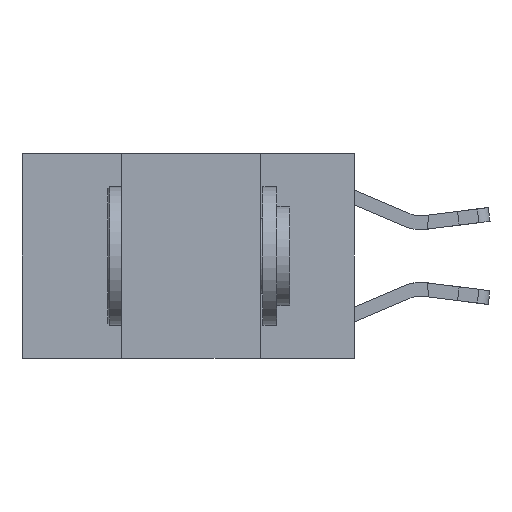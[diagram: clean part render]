
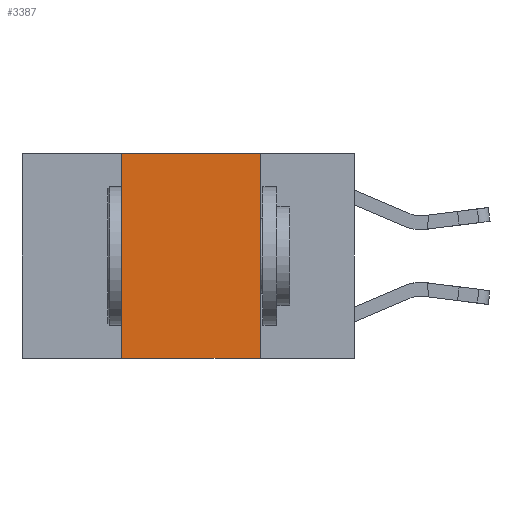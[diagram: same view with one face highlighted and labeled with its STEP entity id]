
A CAD part, left-side view. The second image highlights one B-rep face of the part: STEP entity #3387.
In plain terms, the highlighted planar face has unit normal (-1, 0, 0).
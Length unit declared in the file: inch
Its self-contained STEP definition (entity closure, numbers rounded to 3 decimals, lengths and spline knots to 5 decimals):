
#477 = VERTEX_POINT ( 'NONE', #1706 ) ;
#646 = EDGE_CURVE ( 'NONE', #9966, #10635, #1362, .T. ) ;
#949 = EDGE_CURVE ( 'NONE', #477, #2112, #10585, .T. ) ;
#1362 = LINE ( 'NONE', #8092, #7666 ) ;
#1706 = CARTESIAN_POINT ( 'NONE',  ( 0., 0.17, 0. ) ) ;
#1920 = CARTESIAN_POINT ( 'NONE',  ( 0., 0.6, -0.37 ) ) ;
#1939 = VECTOR ( 'NONE', #5549, 39.37008 ) ;
#2112 = VERTEX_POINT ( 'NONE', #10304 ) ;
#2178 = EDGE_CURVE ( 'NONE', #10635, #477, #13359, .T. ) ;
#2293 = LINE ( 'NONE', #1920, #1939 ) ;
#3252 = AXIS2_PLACEMENT_3D ( 'NONE', #7970, #13397, #6869 ) ;
#3387 = ADVANCED_FACE ( 'NONE', ( #7974 ), #5745, .F. ) ;
#4609 = CARTESIAN_POINT ( 'NONE',  ( 0., 0.42, -0.37 ) ) ;
#5238 = ORIENTED_EDGE ( 'NONE', *, *, #7567, .T. ) ;
#5549 = DIRECTION ( 'NONE',  ( 0., -1., 0. ) ) ;
#5692 = VECTOR ( 'NONE', #5843, 39.37008 ) ;
#5745 = PLANE ( 'NONE',  #3252 ) ;
#5843 = DIRECTION ( 'NONE',  ( 0., 0., -1. ) ) ;
#6869 = DIRECTION ( 'NONE',  ( 0., 0., -1. ) ) ;
#7567 = EDGE_CURVE ( 'NONE', #9966, #2112, #2293, .T. ) ;
#7666 = VECTOR ( 'NONE', #8323, 39.37008 ) ;
#7970 = CARTESIAN_POINT ( 'NONE',  ( 0., 0.6, 0. ) ) ;
#7974 = FACE_OUTER_BOUND ( 'NONE', #13854, .T. ) ;
#8092 = CARTESIAN_POINT ( 'NONE',  ( 0., 0.42, 0. ) ) ;
#8323 = DIRECTION ( 'NONE',  ( 0., 0., 1. ) ) ;
#9466 = ORIENTED_EDGE ( 'NONE', *, *, #646, .F. ) ;
#9500 = CARTESIAN_POINT ( 'NONE',  ( 0., 0.17, 0. ) ) ;
#9966 = VERTEX_POINT ( 'NONE', #4609 ) ;
#10304 = CARTESIAN_POINT ( 'NONE',  ( 0., 0.17, -0.37 ) ) ;
#10547 = VECTOR ( 'NONE', #12712, 39.37008 ) ;
#10584 = CARTESIAN_POINT ( 'NONE',  ( 0., 0.6, 0. ) ) ;
#10585 = LINE ( 'NONE', #9500, #5692 ) ;
#10635 = VERTEX_POINT ( 'NONE', #11976 ) ;
#11955 = ORIENTED_EDGE ( 'NONE', *, *, #949, .F. ) ;
#11976 = CARTESIAN_POINT ( 'NONE',  ( 0., 0.42, 0. ) ) ;
#12435 = ORIENTED_EDGE ( 'NONE', *, *, #2178, .F. ) ;
#12712 = DIRECTION ( 'NONE',  ( 0., -1., 0. ) ) ;
#13359 = LINE ( 'NONE', #10584, #10547 ) ;
#13397 = DIRECTION ( 'NONE',  ( 1., 0., 0. ) ) ;
#13854 = EDGE_LOOP ( 'NONE', ( #11955, #12435, #9466, #5238 ) ) ;
